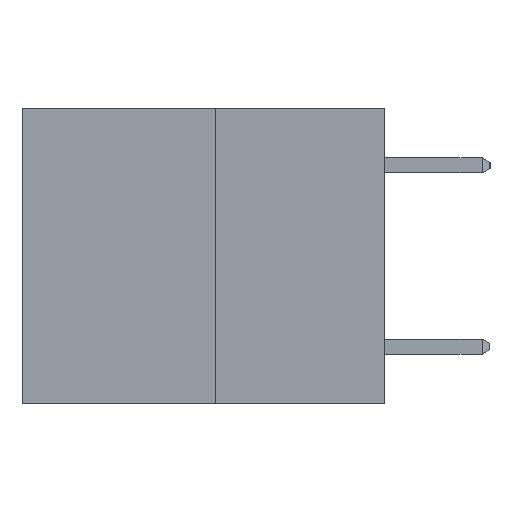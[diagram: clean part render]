
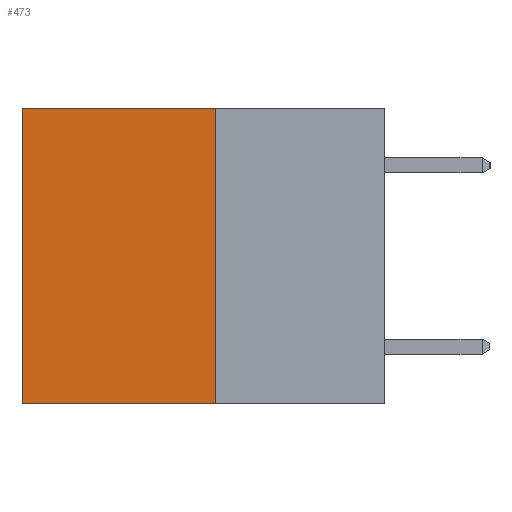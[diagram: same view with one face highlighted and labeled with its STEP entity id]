
A CAD part, left-side view. The second image highlights one B-rep face of the part: STEP entity #473.
In plain terms, the highlighted planar face has unit normal (-1, 0, 0).
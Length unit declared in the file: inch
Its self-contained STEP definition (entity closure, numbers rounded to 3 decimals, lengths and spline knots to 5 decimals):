
#34 = DIRECTION ( 'NONE',  ( 0., 1., 0. ) ) ;
#473 = ADVANCED_FACE ( 'NONE', ( #569 ), #7611, .F. ) ;
#515 = LINE ( 'NONE', #9344, #7955 ) ;
#569 = FACE_OUTER_BOUND ( 'NONE', #3247, .T. ) ;
#1111 = CARTESIAN_POINT ( 'NONE',  ( 0.3165, 0.6, -0.49 ) ) ;
#1241 = ORIENTED_EDGE ( 'NONE', *, *, #6336, .T. ) ;
#1402 = LINE ( 'NONE', #3076, #2396 ) ;
#1560 = VECTOR ( 'NONE', #9488, 39.37008 ) ;
#1903 = CARTESIAN_POINT ( 'NONE',  ( 0.3165, 0.6, 0. ) ) ;
#2153 = VECTOR ( 'NONE', #34, 39.37008 ) ;
#2270 = DIRECTION ( 'NONE',  ( 1., 0., 0. ) ) ;
#2396 = VECTOR ( 'NONE', #4009, 39.37008 ) ;
#2644 = LINE ( 'NONE', #4806, #2153 ) ;
#3076 = CARTESIAN_POINT ( 'NONE',  ( 0.3165, 0.6, -0.49 ) ) ;
#3235 = VERTEX_POINT ( 'NONE', #8753 ) ;
#3247 = EDGE_LOOP ( 'NONE', ( #1241, #8903, #7567, #7205 ) ) ;
#4009 = DIRECTION ( 'NONE',  ( 0., 0., -1. ) ) ;
#4517 = CARTESIAN_POINT ( 'NONE',  ( 0.3165, 0.28, -0.49 ) ) ;
#4806 = CARTESIAN_POINT ( 'NONE',  ( 0.3165, 0.28, -0.49 ) ) ;
#5548 = EDGE_CURVE ( 'NONE', #3235, #9349, #2644, .T. ) ;
#6166 = CARTESIAN_POINT ( 'NONE',  ( 0.3165, 0.28, 0. ) ) ;
#6336 = EDGE_CURVE ( 'NONE', #8107, #9349, #1402, .T. ) ;
#6477 = EDGE_CURVE ( 'NONE', #6849, #8107, #6932, .T. ) ;
#6528 = AXIS2_PLACEMENT_3D ( 'NONE', #4517, #2270, #7588 ) ;
#6849 = VERTEX_POINT ( 'NONE', #6166 ) ;
#6932 = LINE ( 'NONE', #7236, #1560 ) ;
#6966 = DIRECTION ( 'NONE',  ( 0., 0., -1. ) ) ;
#7205 = ORIENTED_EDGE ( 'NONE', *, *, #6477, .T. ) ;
#7236 = CARTESIAN_POINT ( 'NONE',  ( 0.3165, 0.28, 0. ) ) ;
#7567 = ORIENTED_EDGE ( 'NONE', *, *, #7635, .F. ) ;
#7588 = DIRECTION ( 'NONE',  ( 0., 0., -1. ) ) ;
#7611 = PLANE ( 'NONE',  #6528 ) ;
#7635 = EDGE_CURVE ( 'NONE', #6849, #3235, #515, .T. ) ;
#7955 = VECTOR ( 'NONE', #6966, 39.37008 ) ;
#8107 = VERTEX_POINT ( 'NONE', #1903 ) ;
#8753 = CARTESIAN_POINT ( 'NONE',  ( 0.3165, 0.28, -0.49 ) ) ;
#8903 = ORIENTED_EDGE ( 'NONE', *, *, #5548, .F. ) ;
#9344 = CARTESIAN_POINT ( 'NONE',  ( 0.3165, 0.28, -0.49 ) ) ;
#9349 = VERTEX_POINT ( 'NONE', #1111 ) ;
#9488 = DIRECTION ( 'NONE',  ( 0., 1., 0. ) ) ;
